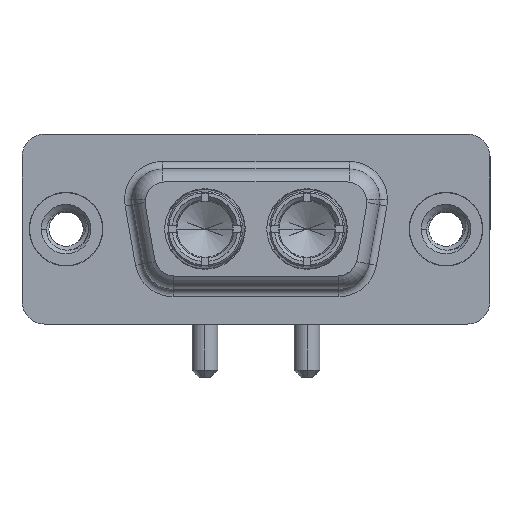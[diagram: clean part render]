
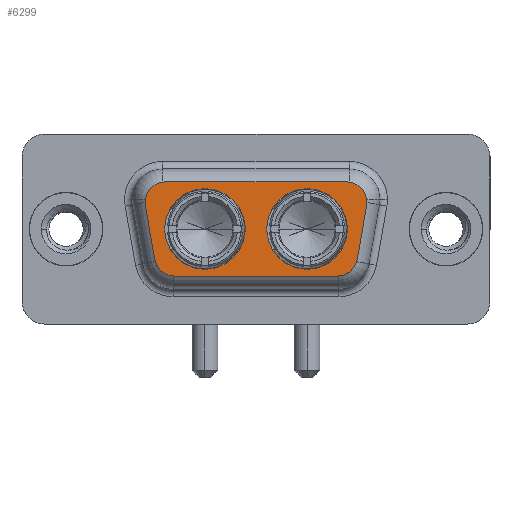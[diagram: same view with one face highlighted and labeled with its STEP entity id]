
A CAD part, top view. The second image highlights one B-rep face of the part: STEP entity #6299.
In plain terms, the highlighted planar face has unit normal (0, 0, 1).
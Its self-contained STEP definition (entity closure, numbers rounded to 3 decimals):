
#120 = VERTEX_POINT ( 'NONE', #535 ) ;
#124 = DIRECTION ( 'NONE',  ( 1., 0., 0. ) ) ;
#129 = DIRECTION ( 'NONE',  ( 1., 0., 0. ) ) ;
#144 = DIRECTION ( 'NONE',  ( 0., 0., 1. ) ) ;
#376 = VECTOR ( 'NONE', #124, 1000. ) ;
#470 = ORIENTED_EDGE ( 'NONE', *, *, #6661, .T. ) ;
#535 = CARTESIAN_POINT ( 'NONE',  ( 19.162, -1.984, 6.2 ) ) ;
#588 = LINE ( 'NONE', #3322, #11628 ) ;
#900 = ORIENTED_EDGE ( 'NONE', *, *, #3604, .F. ) ;
#929 = ORIENTED_EDGE ( 'NONE', *, *, #8459, .F. ) ;
#958 = DIRECTION ( 'NONE',  ( -1., 0., 0. ) ) ;
#1197 = DIRECTION ( 'NONE',  ( 1., 0., 0. ) ) ;
#1251 = CIRCLE ( 'NONE', #2842, 1.35 ) ;
#1375 = EDGE_LOOP ( 'NONE', ( #1896, #929 ) ) ;
#1382 = AXIS2_PLACEMENT_3D ( 'NONE', #1927, #3108, #9527 ) ;
#1400 = EDGE_CURVE ( 'NONE', #3616, #6616, #5969, .T. ) ;
#1467 = CIRCLE ( 'NONE', #9747, 1.35 ) ;
#1491 = DIRECTION ( 'NONE',  ( -1., 0., 0. ) ) ;
#1496 = CARTESIAN_POINT ( 'NONE',  ( 5.2, 1.75, 6.2 ) ) ;
#1602 = CARTESIAN_POINT ( 'NONE',  ( 18.45, 3.1, 6.2 ) ) ;
#1842 = VERTEX_POINT ( 'NONE', #1602 ) ;
#1896 = ORIENTED_EDGE ( 'NONE', *, *, #3654, .F. ) ;
#1927 = CARTESIAN_POINT ( 'NONE',  ( 6.55, 1.75, 6.2 ) ) ;
#2116 = DIRECTION ( 'NONE',  ( 0., 0., -1. ) ) ;
#2147 = EDGE_CURVE ( 'NONE', #120, #4436, #2681, .T. ) ;
#2329 = CIRCLE ( 'NONE', #7083, 2.65 ) ;
#2638 = CIRCLE ( 'NONE', #4424, 2.65 ) ;
#2681 = LINE ( 'NONE', #11319, #5603 ) ;
#2782 = CIRCLE ( 'NONE', #8879, 1.35 ) ;
#2842 = AXIS2_PLACEMENT_3D ( 'NONE', #9952, #4351, #1491 ) ;
#2852 = LINE ( 'NONE', #10256, #10252 ) ;
#3108 = DIRECTION ( 'NONE',  ( 0., 0., 1. ) ) ;
#3112 = ORIENTED_EDGE ( 'NONE', *, *, #12178, .T. ) ;
#3131 = CARTESIAN_POINT ( 'NONE',  ( 11.79, 0., 6.2 ) ) ;
#3135 = CARTESIAN_POINT ( 'NONE',  ( 5.221, 1.516, 6.2 ) ) ;
#3243 = EDGE_LOOP ( 'NONE', ( #4603, #6973, #10441, #10791, #3112, #7579, #9269, #470, #9202 ) ) ;
#3322 = CARTESIAN_POINT ( 'NONE',  ( 5.838, -1.984, 6.2 ) ) ;
#3495 = CARTESIAN_POINT ( 'NONE',  ( 7.167, -1.75, 6.2 ) ) ;
#3604 = EDGE_CURVE ( 'NONE', #4913, #5291, #2329, .T. ) ;
#3616 = VERTEX_POINT ( 'NONE', #6758 ) ;
#3654 = EDGE_CURVE ( 'NONE', #12035, #9889, #7234, .T. ) ;
#3891 = EDGE_CURVE ( 'NONE', #1842, #9037, #2852, .T. ) ;
#4001 = AXIS2_PLACEMENT_3D ( 'NONE', #8454, #6440, #7237 ) ;
#4010 = CARTESIAN_POINT ( 'NONE',  ( 19.779, 1.516, 6.2 ) ) ;
#4351 = DIRECTION ( 'NONE',  ( 0., 0., 1. ) ) ;
#4375 = DIRECTION ( 'NONE',  ( -1., 0., 0. ) ) ;
#4424 = AXIS2_PLACEMENT_3D ( 'NONE', #5926, #144, #1197 ) ;
#4436 = VERTEX_POINT ( 'NONE', #4010 ) ;
#4603 = ORIENTED_EDGE ( 'NONE', *, *, #6461, .T. ) ;
#4812 = PLANE ( 'NONE',  #9653 ) ;
#4913 = VERTEX_POINT ( 'NONE', #3131 ) ;
#4929 = FACE_BOUND ( 'NONE', #1375, .T. ) ;
#5036 = DIRECTION ( 'NONE',  ( 0., 0., 1. ) ) ;
#5127 = EDGE_CURVE ( 'NONE', #11915, #9090, #588, .T. ) ;
#5209 = DIRECTION ( 'NONE',  ( 1., 0., 0. ) ) ;
#5291 = VERTEX_POINT ( 'NONE', #5446 ) ;
#5446 = CARTESIAN_POINT ( 'NONE',  ( 6.49, 0., 6.2 ) ) ;
#5505 = VERTEX_POINT ( 'NONE', #1496 ) ;
#5603 = VECTOR ( 'NONE', #10267, 1000. ) ;
#5926 = CARTESIAN_POINT ( 'NONE',  ( 9.14, 0., 6.2 ) ) ;
#5969 = LINE ( 'NONE', #10559, #376 ) ;
#6299 = ADVANCED_FACE ( 'NONE', ( #4929, #11399, #7645 ), #4812, .F. ) ;
#6440 = DIRECTION ( 'NONE',  ( 0., 0., 1. ) ) ;
#6461 = EDGE_CURVE ( 'NONE', #9090, #3616, #2782, .T. ) ;
#6616 = VERTEX_POINT ( 'NONE', #10094 ) ;
#6661 = EDGE_CURVE ( 'NONE', #5505, #11915, #9076, .T. ) ;
#6665 = CARTESIAN_POINT ( 'NONE',  ( 18.45, 1.75, 6.2 ) ) ;
#6758 = CARTESIAN_POINT ( 'NONE',  ( 7.167, -3.1, 6.2 ) ) ;
#6821 = CARTESIAN_POINT ( 'NONE',  ( 9.14, 0., 6.2 ) ) ;
#6973 = ORIENTED_EDGE ( 'NONE', *, *, #1400, .T. ) ;
#7005 = AXIS2_PLACEMENT_3D ( 'NONE', #9876, #7913, #5209 ) ;
#7083 = AXIS2_PLACEMENT_3D ( 'NONE', #6821, #7801, #129 ) ;
#7234 = CIRCLE ( 'NONE', #11358, 2.65 ) ;
#7237 = DIRECTION ( 'NONE',  ( 1., 0., 0. ) ) ;
#7579 = ORIENTED_EDGE ( 'NONE', *, *, #3891, .T. ) ;
#7645 = FACE_OUTER_BOUND ( 'NONE', #3243, .T. ) ;
#7801 = DIRECTION ( 'NONE',  ( 0., 0., 1. ) ) ;
#7881 = CARTESIAN_POINT ( 'NONE',  ( 7.167, -1.75, 6.2 ) ) ;
#7913 = DIRECTION ( 'NONE',  ( 0., 0., 1. ) ) ;
#8454 = CARTESIAN_POINT ( 'NONE',  ( 15.86, 0., 6.2 ) ) ;
#8459 = EDGE_CURVE ( 'NONE', #9889, #12035, #10107, .T. ) ;
#8879 = AXIS2_PLACEMENT_3D ( 'NONE', #3495, #11018, #4375 ) ;
#9037 = VERTEX_POINT ( 'NONE', #11959 ) ;
#9076 = CIRCLE ( 'NONE', #1382, 1.35 ) ;
#9090 = VERTEX_POINT ( 'NONE', #9177 ) ;
#9138 = DIRECTION ( 'NONE',  ( -1., 0., 0. ) ) ;
#9177 = CARTESIAN_POINT ( 'NONE',  ( 5.838, -1.984, 6.2 ) ) ;
#9202 = ORIENTED_EDGE ( 'NONE', *, *, #5127, .T. ) ;
#9259 = ORIENTED_EDGE ( 'NONE', *, *, #10635, .F. ) ;
#9269 = ORIENTED_EDGE ( 'NONE', *, *, #11600, .T. ) ;
#9527 = DIRECTION ( 'NONE',  ( 1., 0., 0. ) ) ;
#9543 = CIRCLE ( 'NONE', #7005, 1.35 ) ;
#9653 = AXIS2_PLACEMENT_3D ( 'NONE', #7881, #2116, #11646 ) ;
#9747 = AXIS2_PLACEMENT_3D ( 'NONE', #6665, #11166, #958 ) ;
#9854 = DIRECTION ( 'NONE',  ( 0.174, -0.985, 0. ) ) ;
#9876 = CARTESIAN_POINT ( 'NONE',  ( 6.55, 1.75, 6.2 ) ) ;
#9889 = VERTEX_POINT ( 'NONE', #10628 ) ;
#9952 = CARTESIAN_POINT ( 'NONE',  ( 17.833, -1.75, 6.2 ) ) ;
#10094 = CARTESIAN_POINT ( 'NONE',  ( 17.833, -3.1, 6.2 ) ) ;
#10106 = EDGE_CURVE ( 'NONE', #6616, #120, #1251, .T. ) ;
#10107 = CIRCLE ( 'NONE', #4001, 2.65 ) ;
#10252 = VECTOR ( 'NONE', #9138, 1000. ) ;
#10256 = CARTESIAN_POINT ( 'NONE',  ( 6.55, 3.1, 6.2 ) ) ;
#10267 = DIRECTION ( 'NONE',  ( 0.174, 0.985, 0. ) ) ;
#10441 = ORIENTED_EDGE ( 'NONE', *, *, #10106, .T. ) ;
#10559 = CARTESIAN_POINT ( 'NONE',  ( 17.833, -3.1, 6.2 ) ) ;
#10563 = CARTESIAN_POINT ( 'NONE',  ( 15.86, 0., 6.2 ) ) ;
#10628 = CARTESIAN_POINT ( 'NONE',  ( 13.21, 0., 6.2 ) ) ;
#10635 = EDGE_CURVE ( 'NONE', #5291, #4913, #2638, .T. ) ;
#10791 = ORIENTED_EDGE ( 'NONE', *, *, #2147, .T. ) ;
#10852 = CARTESIAN_POINT ( 'NONE',  ( 18.51, 0., 6.2 ) ) ;
#11018 = DIRECTION ( 'NONE',  ( 0., 0., 1. ) ) ;
#11166 = DIRECTION ( 'NONE',  ( 0., 0., 1. ) ) ;
#11319 = CARTESIAN_POINT ( 'NONE',  ( 19.779, 1.516, 6.2 ) ) ;
#11358 = AXIS2_PLACEMENT_3D ( 'NONE', #10563, #5036, #11500 ) ;
#11399 = FACE_BOUND ( 'NONE', #11583, .T. ) ;
#11500 = DIRECTION ( 'NONE',  ( 1., 0., 0. ) ) ;
#11583 = EDGE_LOOP ( 'NONE', ( #900, #9259 ) ) ;
#11600 = EDGE_CURVE ( 'NONE', #9037, #5505, #9543, .T. ) ;
#11628 = VECTOR ( 'NONE', #9854, 1000. ) ;
#11646 = DIRECTION ( 'NONE',  ( -1., 0., 0. ) ) ;
#11915 = VERTEX_POINT ( 'NONE', #3135 ) ;
#11959 = CARTESIAN_POINT ( 'NONE',  ( 6.55, 3.1, 6.2 ) ) ;
#12035 = VERTEX_POINT ( 'NONE', #10852 ) ;
#12178 = EDGE_CURVE ( 'NONE', #4436, #1842, #1467, .T. ) ;
